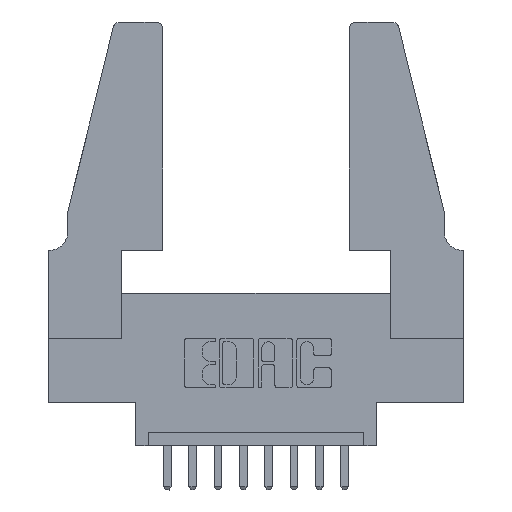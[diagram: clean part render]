
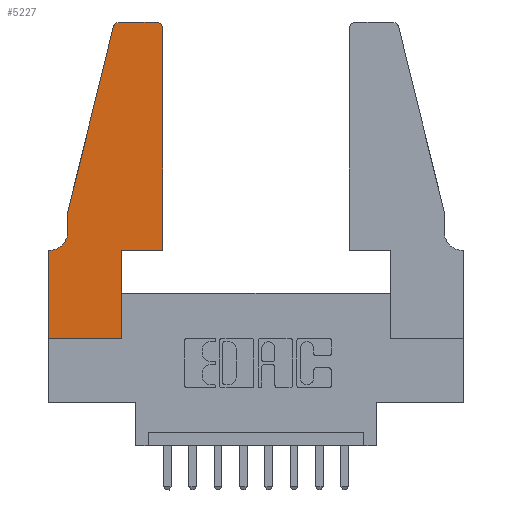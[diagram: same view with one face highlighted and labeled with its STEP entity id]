
A CAD part, top view. The second image highlights one B-rep face of the part: STEP entity #5227.
In plain terms, the highlighted planar face has unit normal (0, 0, 1).
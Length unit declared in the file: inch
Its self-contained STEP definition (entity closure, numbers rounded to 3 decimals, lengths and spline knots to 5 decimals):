
#108 = DIRECTION ( 'NONE',  ( 0., -1., 0. ) ) ;
#152 = CARTESIAN_POINT ( 'NONE',  ( 0.4505, 0.35, 0.37 ) ) ;
#316 = EDGE_CURVE ( 'NONE', #3745, #5198, #5286, .T. ) ;
#412 = CARTESIAN_POINT ( 'NONE',  ( 0.4205, 1.22, 0.37 ) ) ;
#455 = CARTESIAN_POINT ( 'NONE',  ( 0.2865, 0.35, 0.37 ) ) ;
#474 = CARTESIAN_POINT ( 'NONE',  ( 0.284, 1.22, 0.37 ) ) ;
#479 = ORIENTED_EDGE ( 'NONE', *, *, #11221, .T. ) ;
#804 = VERTEX_POINT ( 'NONE', #2472 ) ;
#812 = AXIS2_PLACEMENT_3D ( 'NONE', #412, #12412, #5315 ) ;
#1058 = VECTOR ( 'NONE', #10377, 39.37008 ) ;
#1163 = VERTEX_POINT ( 'NONE', #11719 ) ;
#1166 = CIRCLE ( 'NONE', #5476, 0.07 ) ;
#1188 = DIRECTION ( 'NONE',  ( 0., -1., 0. ) ) ;
#1310 = CARTESIAN_POINT ( 'NONE',  ( 0.25487, 1.22718, 0.37 ) ) ;
#1360 = VECTOR ( 'NONE', #108, 39.37008 ) ;
#1440 = LINE ( 'NONE', #1868, #9330 ) ;
#1574 = CARTESIAN_POINT ( 'NONE',  ( 0.4505, 0.35, 0.37 ) ) ;
#1652 = VECTOR ( 'NONE', #8739, 39.37008 ) ;
#1705 = CARTESIAN_POINT ( 'NONE',  ( 0.2605, 1.25, 0.37 ) ) ;
#1707 = VERTEX_POINT ( 'NONE', #3620 ) ;
#1868 = CARTESIAN_POINT ( 'NONE',  ( 0.0755, 0.35, 0.37 ) ) ;
#1973 = PLANE ( 'NONE',  #8374 ) ;
#2000 = CARTESIAN_POINT ( 'NONE',  ( 0.0055, 0.42, 0.37 ) ) ;
#2231 = EDGE_CURVE ( 'NONE', #2570, #8612, #1166, .T. ) ;
#2468 = DIRECTION ( 'NONE',  ( 1., 0., 0. ) ) ;
#2472 = CARTESIAN_POINT ( 'NONE',  ( 0.284, 1.25, 0.37 ) ) ;
#2570 = VERTEX_POINT ( 'NONE', #10067 ) ;
#2989 = DIRECTION ( 'NONE',  ( 1., 0., 0. ) ) ;
#3105 = DIRECTION ( 'NONE',  ( -1., 0., 0. ) ) ;
#3620 = CARTESIAN_POINT ( 'NONE',  ( 0.2865, 0., 0.37 ) ) ;
#3733 = LINE ( 'NONE', #6333, #1058 ) ;
#3745 = VERTEX_POINT ( 'NONE', #1574 ) ;
#4180 = VERTEX_POINT ( 'NONE', #10570 ) ;
#4219 = EDGE_CURVE ( 'NONE', #804, #7501, #8646, .T. ) ;
#4239 = ORIENTED_EDGE ( 'NONE', *, *, #5298, .T. ) ;
#4282 = DIRECTION ( 'NONE',  ( 0., 1., 0. ) ) ;
#4297 = VECTOR ( 'NONE', #9067, 39.37008 ) ;
#4346 = LINE ( 'NONE', #4645, #1652 ) ;
#4376 = FACE_OUTER_BOUND ( 'NONE', #12614, .T. ) ;
#4645 = CARTESIAN_POINT ( 'NONE',  ( 0., 0., 0.37 ) ) ;
#4669 = LINE ( 'NONE', #5416, #6868 ) ;
#4965 = DIRECTION ( 'NONE',  ( 0., 0., 1. ) ) ;
#5031 = DIRECTION ( 'NONE',  ( 0., 0., -1. ) ) ;
#5176 = CARTESIAN_POINT ( 'NONE',  ( 0., 0., 0.37 ) ) ;
#5198 = VERTEX_POINT ( 'NONE', #5854 ) ;
#5227 = ADVANCED_FACE ( 'NONE', ( #4376 ), #1973, .T. ) ;
#5286 = LINE ( 'NONE', #152, #6992 ) ;
#5298 = EDGE_CURVE ( 'NONE', #1707, #12543, #4669, .T. ) ;
#5315 = DIRECTION ( 'NONE',  ( 1., 0., 0. ) ) ;
#5416 = CARTESIAN_POINT ( 'NONE',  ( 0.2865, 0.35, 0.37 ) ) ;
#5418 = ORIENTED_EDGE ( 'NONE', *, *, #2231, .T. ) ;
#5433 = VECTOR ( 'NONE', #1188, 39.37008 ) ;
#5476 = AXIS2_PLACEMENT_3D ( 'NONE', #2000, #5031, #3105 ) ;
#5574 = AXIS2_PLACEMENT_3D ( 'NONE', #474, #10528, #2468 ) ;
#5854 = CARTESIAN_POINT ( 'NONE',  ( 0.4505, 1.22, 0.37 ) ) ;
#5920 = CARTESIAN_POINT ( 'NONE',  ( 0.0755, 0.5, 0.37 ) ) ;
#5982 = VERTEX_POINT ( 'NONE', #10319 ) ;
#6229 = ORIENTED_EDGE ( 'NONE', *, *, #10934, .T. ) ;
#6333 = CARTESIAN_POINT ( 'NONE',  ( 0.4505, 0.35, 0.37 ) ) ;
#6360 = EDGE_CURVE ( 'NONE', #12543, #3745, #3733, .T. ) ;
#6494 = LINE ( 'NONE', #1705, #4297 ) ;
#6666 = ORIENTED_EDGE ( 'NONE', *, *, #4219, .T. ) ;
#6868 = VECTOR ( 'NONE', #4282, 39.37008 ) ;
#6940 = EDGE_CURVE ( 'NONE', #1163, #804, #6494, .T. ) ;
#6961 = EDGE_CURVE ( 'NONE', #5198, #1163, #9950, .T. ) ;
#6973 = DIRECTION ( 'NONE',  ( -0.239, -0.971, 0. ) ) ;
#6982 = CARTESIAN_POINT ( 'NONE',  ( 0., 0.35, 0.37 ) ) ;
#6992 = VECTOR ( 'NONE', #7973, 39.37008 ) ;
#7148 = ORIENTED_EDGE ( 'NONE', *, *, #316, .T. ) ;
#7214 = CARTESIAN_POINT ( 'NONE',  ( 0.0055, 0.35, 0.37 ) ) ;
#7264 = CARTESIAN_POINT ( 'NONE',  ( 0.0755, 0.5, 0.37 ) ) ;
#7328 = ORIENTED_EDGE ( 'NONE', *, *, #6961, .T. ) ;
#7501 = VERTEX_POINT ( 'NONE', #1310 ) ;
#7631 = EDGE_CURVE ( 'NONE', #8612, #4180, #1440, .T. ) ;
#7732 = ORIENTED_EDGE ( 'NONE', *, *, #6940, .T. ) ;
#7973 = DIRECTION ( 'NONE',  ( 0., 1., 0. ) ) ;
#8374 = AXIS2_PLACEMENT_3D ( 'NONE', #6982, #4965, #2989 ) ;
#8612 = VERTEX_POINT ( 'NONE', #7214 ) ;
#8646 = CIRCLE ( 'NONE', #5574, 0.03 ) ;
#8739 = DIRECTION ( 'NONE',  ( 1., 0., 0. ) ) ;
#8890 = ORIENTED_EDGE ( 'NONE', *, *, #7631, .T. ) ;
#8966 = LINE ( 'NONE', #5920, #11645 ) ;
#9056 = DIRECTION ( 'NONE',  ( -1., 0., 0. ) ) ;
#9067 = DIRECTION ( 'NONE',  ( -1., 0., 0. ) ) ;
#9261 = EDGE_CURVE ( 'NONE', #7501, #5982, #8966, .T. ) ;
#9330 = VECTOR ( 'NONE', #9056, 39.37008 ) ;
#9701 = ORIENTED_EDGE ( 'NONE', *, *, #10683, .T. ) ;
#9950 = CIRCLE ( 'NONE', #812, 0.03 ) ;
#10067 = CARTESIAN_POINT ( 'NONE',  ( 0.0755, 0.42, 0.37 ) ) ;
#10319 = CARTESIAN_POINT ( 'NONE',  ( 0.0755, 0.5, 0.37 ) ) ;
#10377 = DIRECTION ( 'NONE',  ( 1., 0., 0. ) ) ;
#10528 = DIRECTION ( 'NONE',  ( 0., 0., 1. ) ) ;
#10570 = CARTESIAN_POINT ( 'NONE',  ( 0., 0.35, 0.37 ) ) ;
#10683 = EDGE_CURVE ( 'NONE', #4180, #10824, #12680, .T. ) ;
#10824 = VERTEX_POINT ( 'NONE', #12447 ) ;
#10934 = EDGE_CURVE ( 'NONE', #10824, #1707, #4346, .T. ) ;
#11221 = EDGE_CURVE ( 'NONE', #5982, #2570, #11897, .T. ) ;
#11645 = VECTOR ( 'NONE', #6973, 39.37008 ) ;
#11719 = CARTESIAN_POINT ( 'NONE',  ( 0.4205, 1.25, 0.37 ) ) ;
#11897 = LINE ( 'NONE', #7264, #5433 ) ;
#12122 = ORIENTED_EDGE ( 'NONE', *, *, #9261, .T. ) ;
#12412 = DIRECTION ( 'NONE',  ( 0., 0., 1. ) ) ;
#12447 = CARTESIAN_POINT ( 'NONE',  ( 0., 0., 0.37 ) ) ;
#12543 = VERTEX_POINT ( 'NONE', #455 ) ;
#12614 = EDGE_LOOP ( 'NONE', ( #7732, #6666, #12122, #479, #5418, #8890, #9701, #6229, #4239, #12931, #7148, #7328 ) ) ;
#12680 = LINE ( 'NONE', #5176, #1360 ) ;
#12931 = ORIENTED_EDGE ( 'NONE', *, *, #6360, .T. ) ;
